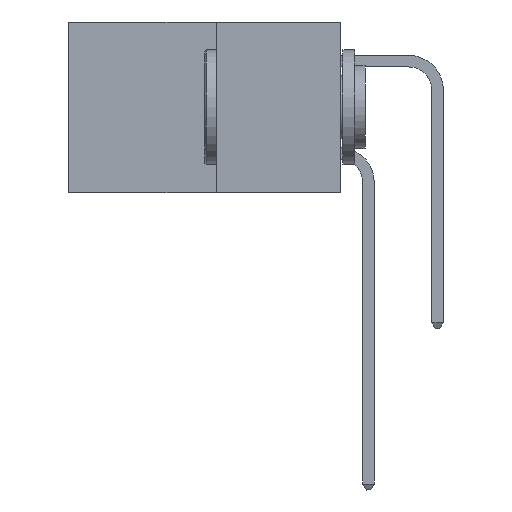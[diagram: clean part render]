
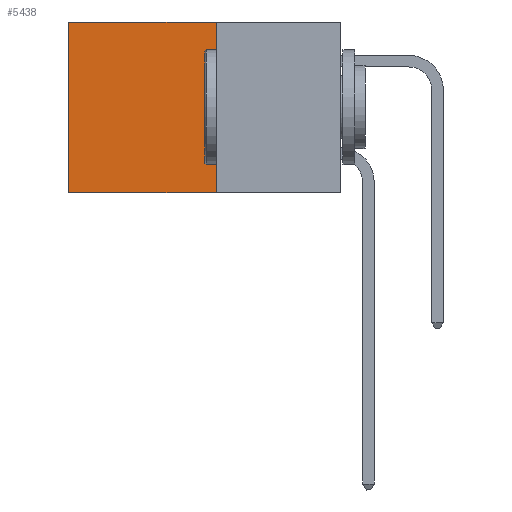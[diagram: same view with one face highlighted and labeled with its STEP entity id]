
A CAD part, left-side view. The second image highlights one B-rep face of the part: STEP entity #5438.
In plain terms, the highlighted planar face has unit normal (-1, 0, 0).
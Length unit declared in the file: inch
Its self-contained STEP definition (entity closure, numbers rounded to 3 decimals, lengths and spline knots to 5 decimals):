
#255 = AXIS2_PLACEMENT_3D ( 'NONE', #13420, #12596, #12529 ) ;
#2613 = FACE_OUTER_BOUND ( 'NONE', #24195, .T. ) ;
#2850 = CARTESIAN_POINT ( 'NONE',  ( 0.277, 0.27, -0.37 ) ) ;
#2900 = EDGE_CURVE ( 'NONE', #12083, #21096, #25895, .T. ) ;
#3040 = DIRECTION ( 'NONE',  ( 0., 1., 0. ) ) ;
#3214 = LINE ( 'NONE', #10121, #15426 ) ;
#3958 = LINE ( 'NONE', #16022, #10042 ) ;
#5438 = ADVANCED_FACE ( 'NONE', ( #2613 ), #12643, .F. ) ;
#6715 = CARTESIAN_POINT ( 'NONE',  ( 0.277, 0.59, -0.37 ) ) ;
#8700 = CARTESIAN_POINT ( 'NONE',  ( 0.277, 0.27, -0.37 ) ) ;
#10042 = VECTOR ( 'NONE', #3040, 39.37008 ) ;
#10061 = ORIENTED_EDGE ( 'NONE', *, *, #2900, .F. ) ;
#10121 = CARTESIAN_POINT ( 'NONE',  ( 0.277, 0.27, -0.37 ) ) ;
#10423 = DIRECTION ( 'NONE',  ( 0., 1., 0. ) ) ;
#12083 = VERTEX_POINT ( 'NONE', #2850 ) ;
#12529 = DIRECTION ( 'NONE',  ( 0., 0., -1. ) ) ;
#12596 = DIRECTION ( 'NONE',  ( 1., 0., 0. ) ) ;
#12643 = PLANE ( 'NONE',  #255 ) ;
#13420 = CARTESIAN_POINT ( 'NONE',  ( 0.277, 0.27, -0.37 ) ) ;
#13840 = CARTESIAN_POINT ( 'NONE',  ( 0.277, 0.59, 0. ) ) ;
#14218 = LINE ( 'NONE', #17473, #19519 ) ;
#14915 = VERTEX_POINT ( 'NONE', #30080 ) ;
#15039 = EDGE_CURVE ( 'NONE', #22561, #21096, #14218, .T. ) ;
#15426 = VECTOR ( 'NONE', #18020, 39.37008 ) ;
#16022 = CARTESIAN_POINT ( 'NONE',  ( 0.277, 0.27, 0. ) ) ;
#17473 = CARTESIAN_POINT ( 'NONE',  ( 0.277, 0.59, -0.37 ) ) ;
#17591 = DIRECTION ( 'NONE',  ( 0., 0., -1. ) ) ;
#18020 = DIRECTION ( 'NONE',  ( 0., 0., -1. ) ) ;
#19519 = VECTOR ( 'NONE', #17591, 39.37008 ) ;
#21096 = VERTEX_POINT ( 'NONE', #6715 ) ;
#21220 = ORIENTED_EDGE ( 'NONE', *, *, #28392, .F. ) ;
#22561 = VERTEX_POINT ( 'NONE', #13840 ) ;
#24195 = EDGE_LOOP ( 'NONE', ( #29051, #10061, #21220, #26343 ) ) ;
#25895 = LINE ( 'NONE', #8700, #31868 ) ;
#26343 = ORIENTED_EDGE ( 'NONE', *, *, #29289, .T. ) ;
#28392 = EDGE_CURVE ( 'NONE', #14915, #12083, #3214, .T. ) ;
#29051 = ORIENTED_EDGE ( 'NONE', *, *, #15039, .T. ) ;
#29289 = EDGE_CURVE ( 'NONE', #14915, #22561, #3958, .T. ) ;
#30080 = CARTESIAN_POINT ( 'NONE',  ( 0.277, 0.27, 0. ) ) ;
#31868 = VECTOR ( 'NONE', #10423, 39.37008 ) ;
